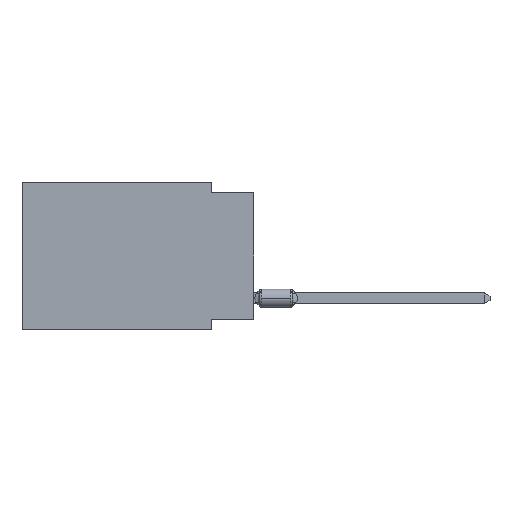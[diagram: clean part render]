
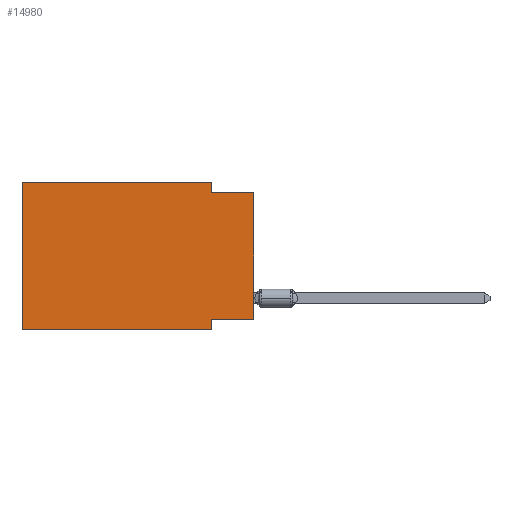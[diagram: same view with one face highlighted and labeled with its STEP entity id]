
A CAD part, left-side view. The second image highlights one B-rep face of the part: STEP entity #14980.
In plain terms, the highlighted planar face has unit normal (-1, 0, 0).
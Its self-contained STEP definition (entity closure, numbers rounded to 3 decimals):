
#249 = EDGE_CURVE ( 'NONE', #1441, #4600, #4381, .T. ) ;
#780 = VERTEX_POINT ( 'NONE', #6837 ) ;
#830 = EDGE_CURVE ( 'NONE', #3548, #2772, #2232, .T. ) ;
#886 = LINE ( 'NONE', #12353, #9655 ) ;
#1171 = CARTESIAN_POINT ( 'NONE',  ( 0., 13.97, -8.89 ) ) ;
#1441 = VERTEX_POINT ( 'NONE', #5594 ) ;
#1591 = CARTESIAN_POINT ( 'NONE',  ( 0., 0., -0.635 ) ) ;
#2232 = LINE ( 'NONE', #6080, #6581 ) ;
#2467 = EDGE_CURVE ( 'NONE', #7012, #4600, #9636, .T. ) ;
#2772 = VERTEX_POINT ( 'NONE', #11522 ) ;
#2823 = VECTOR ( 'NONE', #3773, 1000. ) ;
#3294 = VECTOR ( 'NONE', #16205, 1000. ) ;
#3548 = VERTEX_POINT ( 'NONE', #13795 ) ;
#3705 = VECTOR ( 'NONE', #7125, 1000. ) ;
#3745 = EDGE_CURVE ( 'NONE', #7012, #3548, #14625, .T. ) ;
#3773 = DIRECTION ( 'NONE',  ( 0., 0., 1. ) ) ;
#4141 = ORIENTED_EDGE ( 'NONE', *, *, #8923, .F. ) ;
#4381 = LINE ( 'NONE', #14566, #13785 ) ;
#4475 = LINE ( 'NONE', #10109, #3294 ) ;
#4600 = VERTEX_POINT ( 'NONE', #1591 ) ;
#4755 = AXIS2_PLACEMENT_3D ( 'NONE', #6392, #5137, #10226 ) ;
#5137 = DIRECTION ( 'NONE',  ( 1., 0., 0. ) ) ;
#5594 = CARTESIAN_POINT ( 'NONE',  ( 0., 2.54, -0.635 ) ) ;
#5997 = DIRECTION ( 'NONE',  ( 0., 0., -1. ) ) ;
#6080 = CARTESIAN_POINT ( 'NONE',  ( 0., 2.54, -8.89 ) ) ;
#6392 = CARTESIAN_POINT ( 'NONE',  ( 0., 13.97, 0. ) ) ;
#6581 = VECTOR ( 'NONE', #5997, 1000. ) ;
#6837 = CARTESIAN_POINT ( 'NONE',  ( 0., 13.97, 0. ) ) ;
#7012 = VERTEX_POINT ( 'NONE', #15958 ) ;
#7125 = DIRECTION ( 'NONE',  ( 0., 0., 1. ) ) ;
#7174 = DIRECTION ( 'NONE',  ( 0., -1., 0. ) ) ;
#7395 = ORIENTED_EDGE ( 'NONE', *, *, #3745, .F. ) ;
#7563 = EDGE_LOOP ( 'NONE', ( #13091, #12806, #8499, #4141, #12360, #13176, #16025, #7395 ) ) ;
#7566 = EDGE_CURVE ( 'NONE', #10817, #1441, #886, .T. ) ;
#8116 = EDGE_CURVE ( 'NONE', #14089, #2772, #16019, .T. ) ;
#8495 = DIRECTION ( 'NONE',  ( 0., 0., -1. ) ) ;
#8499 = ORIENTED_EDGE ( 'NONE', *, *, #7566, .F. ) ;
#8923 = EDGE_CURVE ( 'NONE', #780, #10817, #4475, .T. ) ;
#9636 = LINE ( 'NONE', #9711, #3705 ) ;
#9655 = VECTOR ( 'NONE', #8495, 1000. ) ;
#9711 = CARTESIAN_POINT ( 'NONE',  ( 0., 0., 0. ) ) ;
#10109 = CARTESIAN_POINT ( 'NONE',  ( 0., 13.97, 0. ) ) ;
#10143 = FACE_OUTER_BOUND ( 'NONE', #7563, .T. ) ;
#10199 = VECTOR ( 'NONE', #7174, 1000. ) ;
#10226 = DIRECTION ( 'NONE',  ( 0., 0., -1. ) ) ;
#10817 = VERTEX_POINT ( 'NONE', #15881 ) ;
#11522 = CARTESIAN_POINT ( 'NONE',  ( 0., 2.54, -8.89 ) ) ;
#12100 = EDGE_CURVE ( 'NONE', #14089, #780, #12796, .T. ) ;
#12113 = DIRECTION ( 'NONE',  ( 0., 1., 0. ) ) ;
#12353 = CARTESIAN_POINT ( 'NONE',  ( 0., 2.54, 0. ) ) ;
#12360 = ORIENTED_EDGE ( 'NONE', *, *, #12100, .F. ) ;
#12753 = PLANE ( 'NONE',  #4755 ) ;
#12796 = LINE ( 'NONE', #16361, #2823 ) ;
#12806 = ORIENTED_EDGE ( 'NONE', *, *, #249, .F. ) ;
#12807 = VECTOR ( 'NONE', #12113, 1000. ) ;
#13076 = DIRECTION ( 'NONE',  ( 0., -1., 0. ) ) ;
#13091 = ORIENTED_EDGE ( 'NONE', *, *, #2467, .T. ) ;
#13176 = ORIENTED_EDGE ( 'NONE', *, *, #8116, .T. ) ;
#13617 = CARTESIAN_POINT ( 'NONE',  ( 0., 13.97, -8.89 ) ) ;
#13785 = VECTOR ( 'NONE', #13076, 1000. ) ;
#13795 = CARTESIAN_POINT ( 'NONE',  ( 0., 2.54, -8.255 ) ) ;
#14089 = VERTEX_POINT ( 'NONE', #1171 ) ;
#14566 = CARTESIAN_POINT ( 'NONE',  ( 0., 0., -0.635 ) ) ;
#14625 = LINE ( 'NONE', #14781, #12807 ) ;
#14781 = CARTESIAN_POINT ( 'NONE',  ( 0., 0., -8.255 ) ) ;
#14980 = ADVANCED_FACE ( 'NONE', ( #10143 ), #12753, .F. ) ;
#15881 = CARTESIAN_POINT ( 'NONE',  ( 0., 2.54, 0. ) ) ;
#15958 = CARTESIAN_POINT ( 'NONE',  ( 0., 0., -8.255 ) ) ;
#16019 = LINE ( 'NONE', #13617, #10199 ) ;
#16025 = ORIENTED_EDGE ( 'NONE', *, *, #830, .F. ) ;
#16205 = DIRECTION ( 'NONE',  ( 0., -1., 0. ) ) ;
#16361 = CARTESIAN_POINT ( 'NONE',  ( 0., 13.97, 0. ) ) ;
